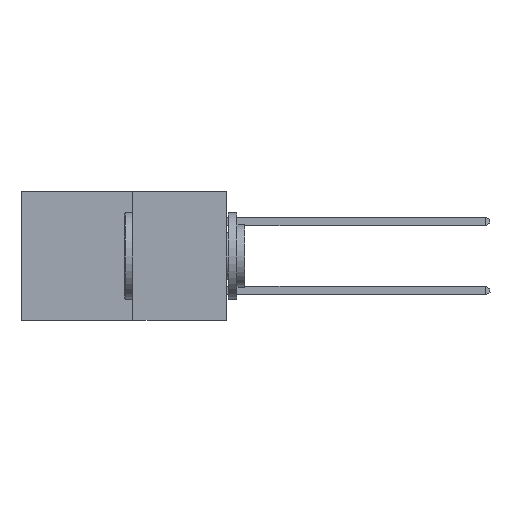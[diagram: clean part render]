
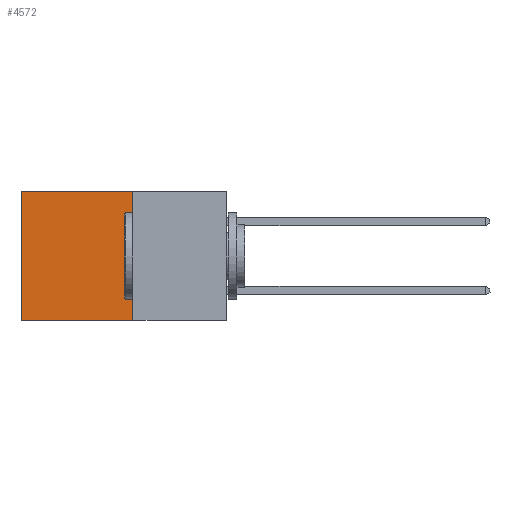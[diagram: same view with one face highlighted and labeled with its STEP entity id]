
A CAD part, left-side view. The second image highlights one B-rep face of the part: STEP entity #4572.
In plain terms, the highlighted planar face has unit normal (-1, 0, 0).
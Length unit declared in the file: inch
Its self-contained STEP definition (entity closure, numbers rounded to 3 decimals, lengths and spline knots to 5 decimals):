
#364 = AXIS2_PLACEMENT_3D ( 'NONE', #28635, #28326, #28253 ) ;
#537 = CARTESIAN_POINT ( 'NONE',  ( 0.277, 0.59, -0.37 ) ) ;
#1114 = EDGE_CURVE ( 'NONE', #20186, #5178, #32238, .T. ) ;
#3806 = ORIENTED_EDGE ( 'NONE', *, *, #1114, .T. ) ;
#4572 = ADVANCED_FACE ( 'NONE', ( #25564 ), #28887, .F. ) ;
#5178 = VERTEX_POINT ( 'NONE', #537 ) ;
#6106 = DIRECTION ( 'NONE',  ( 0., 1., 0. ) ) ;
#6835 = DIRECTION ( 'NONE',  ( 0., 0., -1. ) ) ;
#8190 = EDGE_LOOP ( 'NONE', ( #3806, #24231, #9755, #17802 ) ) ;
#8819 = DIRECTION ( 'NONE',  ( 0., 0., -1. ) ) ;
#9330 = EDGE_CURVE ( 'NONE', #15529, #20186, #18139, .T. ) ;
#9755 = ORIENTED_EDGE ( 'NONE', *, *, #16907, .F. ) ;
#10802 = VECTOR ( 'NONE', #6106, 39.37008 ) ;
#15372 = CARTESIAN_POINT ( 'NONE',  ( 0.277, 0.59, -0.37 ) ) ;
#15529 = VERTEX_POINT ( 'NONE', #27468 ) ;
#16907 = EDGE_CURVE ( 'NONE', #15529, #18821, #26109, .T. ) ;
#17802 = ORIENTED_EDGE ( 'NONE', *, *, #9330, .T. ) ;
#18139 = LINE ( 'NONE', #22858, #23419 ) ;
#18821 = VERTEX_POINT ( 'NONE', #30357 ) ;
#19197 = VECTOR ( 'NONE', #6835, 39.37008 ) ;
#20186 = VERTEX_POINT ( 'NONE', #27617 ) ;
#20758 = DIRECTION ( 'NONE',  ( 0., 1., 0. ) ) ;
#22244 = EDGE_CURVE ( 'NONE', #18821, #5178, #31632, .T. ) ;
#22858 = CARTESIAN_POINT ( 'NONE',  ( 0.277, 0.27, 0. ) ) ;
#23419 = VECTOR ( 'NONE', #20758, 39.37008 ) ;
#24231 = ORIENTED_EDGE ( 'NONE', *, *, #22244, .F. ) ;
#24547 = CARTESIAN_POINT ( 'NONE',  ( 0.277, 0.27, -0.37 ) ) ;
#25564 = FACE_OUTER_BOUND ( 'NONE', #8190, .T. ) ;
#26109 = LINE ( 'NONE', #27867, #19197 ) ;
#27468 = CARTESIAN_POINT ( 'NONE',  ( 0.277, 0.27, 0. ) ) ;
#27617 = CARTESIAN_POINT ( 'NONE',  ( 0.277, 0.59, 0. ) ) ;
#27867 = CARTESIAN_POINT ( 'NONE',  ( 0.277, 0.27, -0.37 ) ) ;
#28253 = DIRECTION ( 'NONE',  ( 0., 0., -1. ) ) ;
#28326 = DIRECTION ( 'NONE',  ( 1., 0., 0. ) ) ;
#28635 = CARTESIAN_POINT ( 'NONE',  ( 0.277, 0.27, -0.37 ) ) ;
#28887 = PLANE ( 'NONE',  #364 ) ;
#30357 = CARTESIAN_POINT ( 'NONE',  ( 0.277, 0.27, -0.37 ) ) ;
#31446 = VECTOR ( 'NONE', #8819, 39.37008 ) ;
#31632 = LINE ( 'NONE', #24547, #10802 ) ;
#32238 = LINE ( 'NONE', #15372, #31446 ) ;
